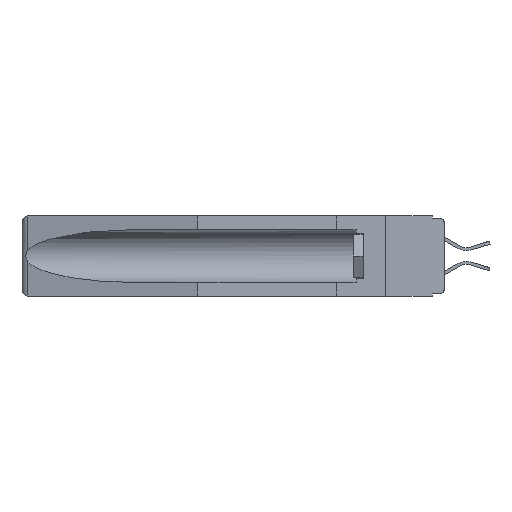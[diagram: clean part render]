
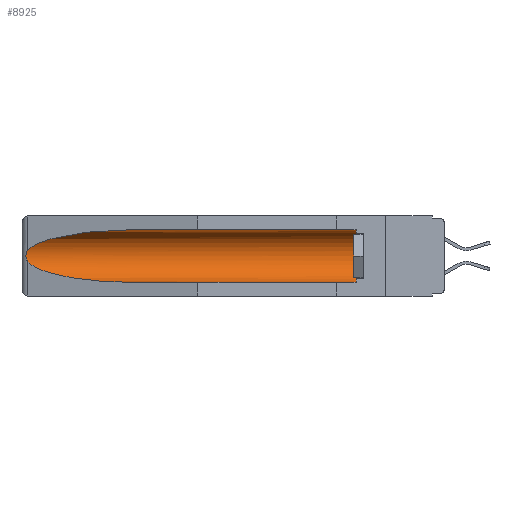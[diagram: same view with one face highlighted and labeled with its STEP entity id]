
A CAD part, left-side view. The second image highlights one B-rep face of the part: STEP entity #8925.
In plain terms, the highlighted cylindrical face has radius 2.857 mm (diameter 5.715 mm), a partial arc.
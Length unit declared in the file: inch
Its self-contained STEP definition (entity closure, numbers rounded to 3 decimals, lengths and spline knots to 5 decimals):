
#15 = VERTEX_POINT ( 'NONE', #8402 ) ;
#373 = DIRECTION ( 'NONE',  ( 0., 1., 0. ) ) ;
#519 = EDGE_CURVE ( 'NONE', #6780, #3801, #14702, .T. ) ;
#818 = EDGE_CURVE ( 'NONE', #3094, #5234, #4119, .T. ) ;
#987 =( BOUNDED_CURVE ( )  B_SPLINE_CURVE ( 3, ( #5444, #1610, #12832, #5284 ),
 .UNSPECIFIED., .F., .F. ) 
 B_SPLINE_CURVE_WITH_KNOTS ( ( 4, 4 ),
 ( 0.1948, 1.5708 ),
 .UNSPECIFIED. ) 
 CURVE ( )  GEOMETRIC_REPRESENTATION_ITEM ( )  RATIONAL_B_SPLINE_CURVE ( ( 1., 0.848, 0.848, 1. ) ) 
 REPRESENTATION_ITEM ( '' )  );
#1068 = CARTESIAN_POINT ( 'NONE',  ( 0.21114, 1.30732, -0.059 ) ) ;
#1149 = CARTESIAN_POINT ( 'NONE',  ( 0.26537, 1.52718, -0.14972 ) ) ;
#1314 = CARTESIAN_POINT ( 'NONE',  ( 0.155, 1.07973, -0.284 ) ) ;
#1317 = CARTESIAN_POINT ( 'NONE',  ( 0.26597, 1.5296, -0.19026 ) ) ;
#1610 = CARTESIAN_POINT ( 'NONE',  ( 0.25451, 1.48313, -0.24835 ) ) ;
#1671 = DIRECTION ( 'NONE',  ( 0., 0., 1. ) ) ;
#1811 = VERTEX_POINT ( 'NONE', #7998 ) ;
#2168 = VECTOR ( 'NONE', #5338, 39.37008 ) ;
#2532 = CARTESIAN_POINT ( 'NONE',  ( 0.2673, 1.5327, -0.16383 ) ) ;
#2608 = CARTESIAN_POINT ( 'NONE',  ( 0.26597, 1.52961, -0.15275 ) ) ;
#3094 = VERTEX_POINT ( 'NONE', #12769 ) ;
#3404 = EDGE_LOOP ( 'NONE', ( #9777, #9582, #3733, #4723, #11128, #13126 ) ) ;
#3661 = CARTESIAN_POINT ( 'NONE',  ( 0.26654, 1.53092, -0.15636 ) ) ;
#3733 = ORIENTED_EDGE ( 'NONE', *, *, #8479, .T. ) ;
#3801 = VERTEX_POINT ( 'NONE', #8777 ) ;
#4119 = LINE ( 'NONE', #8868, #2168 ) ;
#4443 = DIRECTION ( 'NONE',  ( 0., 0., 1. ) ) ;
#4723 = ORIENTED_EDGE ( 'NONE', *, *, #818, .F. ) ;
#5234 = VERTEX_POINT ( 'NONE', #1314 ) ;
#5268 = CYLINDRICAL_SURFACE ( 'NONE', #6889, 0.1125 ) ;
#5284 = CARTESIAN_POINT ( 'NONE',  ( 0.155, 1.07973, -0.284 ) ) ;
#5338 = DIRECTION ( 'NONE',  ( 0., 1., 0. ) ) ;
#5345 = CARTESIAN_POINT ( 'NONE',  ( 0.155, -0.30754, -0.1715 ) ) ;
#5444 = CARTESIAN_POINT ( 'NONE',  ( 0.26537, 1.52718, -0.19328 ) ) ;
#6052 = CARTESIAN_POINT ( 'NONE',  ( 0.2675, 1.53308, -0.16763 ) ) ;
#6633 = EDGE_CURVE ( 'NONE', #15, #1811, #12717, .T. ) ;
#6780 = VERTEX_POINT ( 'NONE', #9156 ) ;
#6889 = AXIS2_PLACEMENT_3D ( 'NONE', #5345, #373, #1671 ) ;
#7258 = CARTESIAN_POINT ( 'NONE',  ( 0.155, -0.30754, -0.059 ) ) ;
#7544 = CARTESIAN_POINT ( 'NONE',  ( 0.2675, 1.53308, -0.17534 ) ) ;
#7998 = CARTESIAN_POINT ( 'NONE',  ( 0.26537, 1.52718, -0.19328 ) ) ;
#8184 =( BOUNDED_CURVE ( )  B_SPLINE_CURVE ( 3, ( #8423, #1068, #13427, #1149 ),
 .UNSPECIFIED., .F., .F. ) 
 B_SPLINE_CURVE_WITH_KNOTS ( ( 4, 4 ),
 ( 4.71239, 6.08839 ),
 .UNSPECIFIED. ) 
 CURVE ( )  GEOMETRIC_REPRESENTATION_ITEM ( )  RATIONAL_B_SPLINE_CURVE ( ( 1., 0.848, 0.848, 1. ) ) 
 REPRESENTATION_ITEM ( '' )  );
#8188 = AXIS2_PLACEMENT_3D ( 'NONE', #8298, #13292, #4443 ) ;
#8298 = CARTESIAN_POINT ( 'NONE',  ( 0.155, 0.126, -0.1715 ) ) ;
#8402 = CARTESIAN_POINT ( 'NONE',  ( 0.26537, 1.52718, -0.14972 ) ) ;
#8423 = CARTESIAN_POINT ( 'NONE',  ( 0.155, 1.07973, -0.059 ) ) ;
#8479 = EDGE_CURVE ( 'NONE', #1811, #5234, #987, .T. ) ;
#8541 = DIRECTION ( 'NONE',  ( 0., 1., 0. ) ) ;
#8777 = CARTESIAN_POINT ( 'NONE',  ( 0.155, 1.07973, -0.059 ) ) ;
#8868 = CARTESIAN_POINT ( 'NONE',  ( 0.155, -0.30754, -0.284 ) ) ;
#8925 = ADVANCED_FACE ( 'NONE', ( #13968 ), #5268, .F. ) ;
#9099 = EDGE_CURVE ( 'NONE', #3094, #6780, #13153, .T. ) ;
#9156 = CARTESIAN_POINT ( 'NONE',  ( 0.155, 0.126, -0.059 ) ) ;
#9582 = ORIENTED_EDGE ( 'NONE', *, *, #6633, .T. ) ;
#9777 = ORIENTED_EDGE ( 'NONE', *, *, #13537, .T. ) ;
#9810 = CARTESIAN_POINT ( 'NONE',  ( 0.2673, 1.53269, -0.17917 ) ) ;
#10426 = VECTOR ( 'NONE', #8541, 39.37008 ) ;
#11128 = ORIENTED_EDGE ( 'NONE', *, *, #9099, .T. ) ;
#12522 = CARTESIAN_POINT ( 'NONE',  ( 0.26655, 1.53094, -0.18657 ) ) ;
#12717 = B_SPLINE_CURVE_WITH_KNOTS ( 'NONE', 3,
 ( #13760, #2608, #3661, #2532, #6052, #7544, #9810, #12522, #1317, #13593 ),
 .UNSPECIFIED., .F., .F.,
 ( 4, 2, 2, 2, 4 ),
 ( 0., 0.00029, 0.00058, 0.00087, 0.00117 ),
 .UNSPECIFIED. ) ;
#12769 = CARTESIAN_POINT ( 'NONE',  ( 0.155, 0.126, -0.284 ) ) ;
#12832 = CARTESIAN_POINT ( 'NONE',  ( 0.21114, 1.30732, -0.284 ) ) ;
#13126 = ORIENTED_EDGE ( 'NONE', *, *, #519, .T. ) ;
#13153 = CIRCLE ( 'NONE', #8188, 0.1125 ) ;
#13292 = DIRECTION ( 'NONE',  ( 0., -1., 0. ) ) ;
#13427 = CARTESIAN_POINT ( 'NONE',  ( 0.25451, 1.48313, -0.09465 ) ) ;
#13537 = EDGE_CURVE ( 'NONE', #3801, #15, #8184, .T. ) ;
#13593 = CARTESIAN_POINT ( 'NONE',  ( 0.26537, 1.52718, -0.19328 ) ) ;
#13760 = CARTESIAN_POINT ( 'NONE',  ( 0.26537, 1.52718, -0.14972 ) ) ;
#13968 = FACE_OUTER_BOUND ( 'NONE', #3404, .T. ) ;
#14702 = LINE ( 'NONE', #7258, #10426 ) ;
